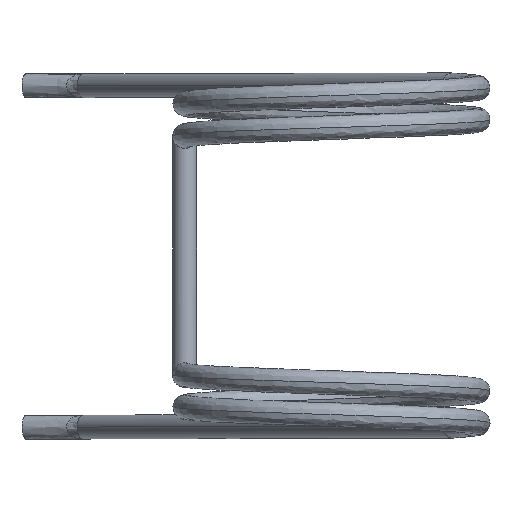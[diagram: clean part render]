
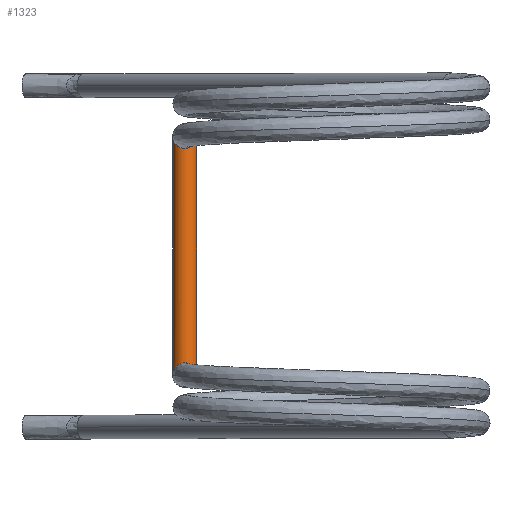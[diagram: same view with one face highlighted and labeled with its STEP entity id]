
A CAD part, top view. The second image highlights one B-rep face of the part: STEP entity #1323.
In plain terms, the highlighted cylindrical face has radius 0.445 mm (diameter 0.889 mm), a partial arc.
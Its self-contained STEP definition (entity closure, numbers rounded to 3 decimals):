
#72 = VECTOR ( 'NONE', #1908, 1000. ) ;
#76 = CARTESIAN_POINT ( 'NONE',  ( 0.445, -0.889, -13.271 ) ) ;
#97 = ORIENTED_EDGE ( 'NONE', *, *, #196, .F. ) ;
#135 = VECTOR ( 'NONE', #1422, 1000. ) ;
#138 = CARTESIAN_POINT ( 'NONE',  ( -0.445, 0., -14.16 ) ) ;
#196 = EDGE_CURVE ( 'NONE', #1859, #901, #1238, .T. ) ;
#198 = CARTESIAN_POINT ( 'NONE',  ( -0.445, -8.001, -13.271 ) ) ;
#260 = ORIENTED_EDGE ( 'NONE', *, *, #419, .F. ) ;
#267 = VERTEX_POINT ( 'NONE', #1828 ) ;
#302 = LINE ( 'NONE', #138, #135 ) ;
#344 = CARTESIAN_POINT ( 'NONE',  ( -0.445, -8.89, -14.161 ) ) ;
#419 = EDGE_CURVE ( 'NONE', #1792, #1859, #1097, .T. ) ;
#464 = DIRECTION ( 'NONE',  ( 0., -1., 0. ) ) ;
#489 = ORIENTED_EDGE ( 'NONE', *, *, #1761, .F. ) ;
#634 = DIRECTION ( 'NONE',  ( 1., 0., 0. ) ) ;
#772 = CARTESIAN_POINT ( 'NONE',  ( 0., 0., -14.16 ) ) ;
#872 = ORIENTED_EDGE ( 'NONE', *, *, #934, .T. ) ;
#901 = VERTEX_POINT ( 'NONE', #1778 ) ;
#904 = CYLINDRICAL_SURFACE ( 'NONE', #2061, 0.445 ) ;
#934 = EDGE_CURVE ( 'NONE', #267, #901, #302, .T. ) ;
#999 = CARTESIAN_POINT ( 'NONE',  ( 0.445, -8.89, -14.161 ) ) ;
#1051 = FACE_OUTER_BOUND ( 'NONE', #2064, .T. ) ;
#1097 = LINE ( 'NONE', #1430, #72 ) ;
#1150 = CARTESIAN_POINT ( 'NONE',  ( 0.445, -8.001, -13.271 ) ) ;
#1238 =( BOUNDED_CURVE ( )  B_SPLINE_CURVE ( 3, ( #999, #1150, #198, #344 ),
 .UNSPECIFIED., .F., .F. ) 
 B_SPLINE_CURVE_WITH_KNOTS ( ( 4, 4 ),
 ( 1.571, 4.712 ),
 .UNSPECIFIED. ) 
 CURVE ( )  GEOMETRIC_REPRESENTATION_ITEM ( )  RATIONAL_B_SPLINE_CURVE ( ( 1., 0.333, 0.333, 1. ) ) 
 REPRESENTATION_ITEM ( '' )  );
#1323 = ADVANCED_FACE ( 'NONE', ( #1051 ), #904, .T. ) ;
#1422 = DIRECTION ( 'NONE',  ( 0., -1., 0. ) ) ;
#1430 = CARTESIAN_POINT ( 'NONE',  ( 0.445, 0., -14.16 ) ) ;
#1701 = CARTESIAN_POINT ( 'NONE',  ( 0.445, 0., -14.161 ) ) ;
#1712 = CARTESIAN_POINT ( 'NONE',  ( 0.445, 0., -14.161 ) ) ;
#1741 = CARTESIAN_POINT ( 'NONE',  ( 0.445, -8.89, -14.161 ) ) ;
#1761 = EDGE_CURVE ( 'NONE', #267, #1792, #1893, .T. ) ;
#1778 = CARTESIAN_POINT ( 'NONE',  ( -0.445, -8.89, -14.161 ) ) ;
#1792 = VERTEX_POINT ( 'NONE', #1701 ) ;
#1828 = CARTESIAN_POINT ( 'NONE',  ( -0.445, 0., -14.161 ) ) ;
#1859 = VERTEX_POINT ( 'NONE', #1741 ) ;
#1866 = CARTESIAN_POINT ( 'NONE',  ( -0.445, 0., -14.161 ) ) ;
#1893 =( BOUNDED_CURVE ( )  B_SPLINE_CURVE ( 3, ( #1866, #2036, #76, #1712 ),
 .UNSPECIFIED., .F., .F. ) 
 B_SPLINE_CURVE_WITH_KNOTS ( ( 4, 4 ),
 ( 1.571, 4.712 ),
 .UNSPECIFIED. ) 
 CURVE ( )  GEOMETRIC_REPRESENTATION_ITEM ( )  RATIONAL_B_SPLINE_CURVE ( ( 1., 0.333, 0.333, 1. ) ) 
 REPRESENTATION_ITEM ( '' )  );
#1908 = DIRECTION ( 'NONE',  ( 0., -1., 0. ) ) ;
#2036 = CARTESIAN_POINT ( 'NONE',  ( -0.445, -0.889, -13.271 ) ) ;
#2061 = AXIS2_PLACEMENT_3D ( 'NONE', #772, #464, #634 ) ;
#2064 = EDGE_LOOP ( 'NONE', ( #489, #872, #97, #260 ) ) ;
